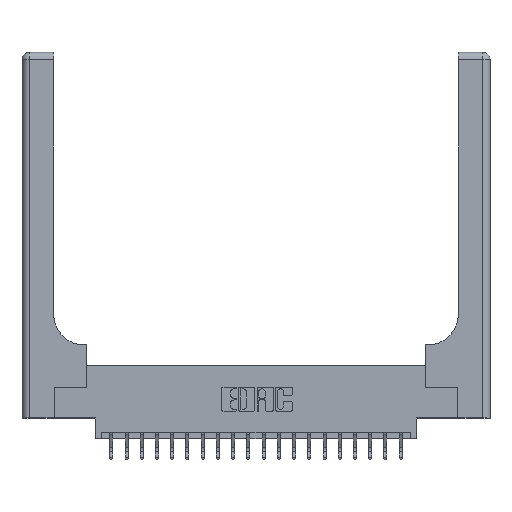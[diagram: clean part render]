
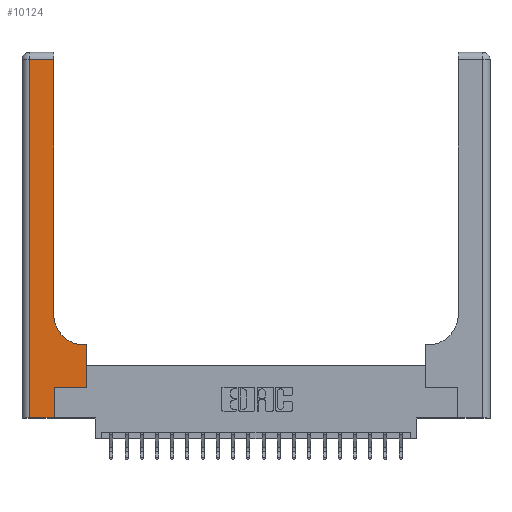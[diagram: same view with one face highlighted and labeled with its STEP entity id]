
A CAD part, top view. The second image highlights one B-rep face of the part: STEP entity #10124.
In plain terms, the highlighted planar face has unit normal (0, 0, 1).
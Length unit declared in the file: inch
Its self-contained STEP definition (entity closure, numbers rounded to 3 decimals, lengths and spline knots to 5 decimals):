
#57 = VERTEX_POINT ( 'NONE', #2765 ) ;
#139 = CARTESIAN_POINT ( 'NONE',  ( 0.528, 0.6, 0.37 ) ) ;
#674 = CIRCLE ( 'NONE', #13136, 0.25 ) ;
#698 = ORIENTED_EDGE ( 'NONE', *, *, #1223, .T. ) ;
#932 = ORIENTED_EDGE ( 'NONE', *, *, #13584, .T. ) ;
#1223 = EDGE_CURVE ( 'NONE', #16627, #3010, #13035, .T. ) ;
#1424 = CARTESIAN_POINT ( 'NONE',  ( 0.26, 0.6, 0.37 ) ) ;
#1683 = CARTESIAN_POINT ( 'NONE',  ( 0.51, 0.85, 0.37 ) ) ;
#1920 = VERTEX_POINT ( 'NONE', #8875 ) ;
#2040 = VECTOR ( 'NONE', #5160, 39.37008 ) ;
#2052 = LINE ( 'NONE', #10752, #2040 ) ;
#2426 = VERTEX_POINT ( 'NONE', #19408 ) ;
#2433 = CARTESIAN_POINT ( 'NONE',  ( 0.265, 0., 0.37 ) ) ;
#2642 = VERTEX_POINT ( 'NONE', #139 ) ;
#2765 = CARTESIAN_POINT ( 'NONE',  ( 0.265, 0., 0.37 ) ) ;
#2771 = ORIENTED_EDGE ( 'NONE', *, *, #15259, .T. ) ;
#2791 = LINE ( 'NONE', #13460, #11475 ) ;
#2866 = LINE ( 'NONE', #1424, #13547 ) ;
#3010 = VERTEX_POINT ( 'NONE', #9829 ) ;
#3106 = EDGE_CURVE ( 'NONE', #17928, #1920, #674, .T. ) ;
#3261 = EDGE_CURVE ( 'NONE', #13300, #2426, #14153, .T. ) ;
#3462 = EDGE_LOOP ( 'NONE', ( #14920, #10365, #698, #2771, #932, #14334, #10957, #6862, #9810 ) ) ;
#4214 = CARTESIAN_POINT ( 'NONE',  ( 0.528, 0.25, 0.37 ) ) ;
#4357 = DIRECTION ( 'NONE',  ( 0., 1., 0. ) ) ;
#4392 = EDGE_CURVE ( 'NONE', #2426, #2642, #17804, .T. ) ;
#5160 = DIRECTION ( 'NONE',  ( -1., 0., 0. ) ) ;
#5792 = DIRECTION ( 'NONE',  ( 0., 1., 0. ) ) ;
#6024 = LINE ( 'NONE', #7929, #8051 ) ;
#6564 = PLANE ( 'NONE',  #13225 ) ;
#6577 = CARTESIAN_POINT ( 'NONE',  ( 0.51, 0.6, 0.37 ) ) ;
#6862 = ORIENTED_EDGE ( 'NONE', *, *, #6983, .T. ) ;
#6983 = EDGE_CURVE ( 'NONE', #2642, #17928, #2866, .T. ) ;
#7684 = DIRECTION ( 'NONE',  ( 1., 0., 0. ) ) ;
#7822 = VECTOR ( 'NONE', #7684, 39.37008 ) ;
#7929 = CARTESIAN_POINT ( 'NONE',  ( 0., 0., 0.37 ) ) ;
#8051 = VECTOR ( 'NONE', #11399, 39.37008 ) ;
#8203 = EDGE_CURVE ( 'NONE', #1920, #18540, #2791, .T. ) ;
#8726 = VECTOR ( 'NONE', #5792, 39.37008 ) ;
#8742 = CARTESIAN_POINT ( 'NONE',  ( 0.26, 2.94, 0.37 ) ) ;
#8875 = CARTESIAN_POINT ( 'NONE',  ( 0.26, 0.85, 0.37 ) ) ;
#9143 = DIRECTION ( 'NONE',  ( 0., 1., 0. ) ) ;
#9810 = ORIENTED_EDGE ( 'NONE', *, *, #3106, .T. ) ;
#9829 = CARTESIAN_POINT ( 'NONE',  ( 0.06, 0., 0.37 ) ) ;
#10124 = ADVANCED_FACE ( 'NONE', ( #15340 ), #6564, .F. ) ;
#10250 = DIRECTION ( 'NONE',  ( 0., 0., -1. ) ) ;
#10365 = ORIENTED_EDGE ( 'NONE', *, *, #18594, .T. ) ;
#10752 = CARTESIAN_POINT ( 'NONE',  ( 0., 2.94, 0.37 ) ) ;
#10957 = ORIENTED_EDGE ( 'NONE', *, *, #4392, .T. ) ;
#11253 = VECTOR ( 'NONE', #9143, 39.37008 ) ;
#11399 = DIRECTION ( 'NONE',  ( 1., 0., 0. ) ) ;
#11475 = VECTOR ( 'NONE', #4357, 39.37008 ) ;
#11596 = DIRECTION ( 'NONE',  ( -1., 0., 0. ) ) ;
#13035 = LINE ( 'NONE', #16474, #18280 ) ;
#13136 = AXIS2_PLACEMENT_3D ( 'NONE', #1683, #13602, #20487 ) ;
#13225 = AXIS2_PLACEMENT_3D ( 'NONE', #13359, #10250, #11596 ) ;
#13300 = VERTEX_POINT ( 'NONE', #18155 ) ;
#13359 = CARTESIAN_POINT ( 'NONE',  ( 0., 3., 0.37 ) ) ;
#13460 = CARTESIAN_POINT ( 'NONE',  ( 0.26, 3., 0.37 ) ) ;
#13547 = VECTOR ( 'NONE', #19792, 39.37008 ) ;
#13584 = EDGE_CURVE ( 'NONE', #57, #13300, #20920, .T. ) ;
#13602 = DIRECTION ( 'NONE',  ( 0., 0., -1. ) ) ;
#14153 = LINE ( 'NONE', #21243, #7822 ) ;
#14334 = ORIENTED_EDGE ( 'NONE', *, *, #3261, .T. ) ;
#14920 = ORIENTED_EDGE ( 'NONE', *, *, #8203, .T. ) ;
#15259 = EDGE_CURVE ( 'NONE', #3010, #57, #6024, .T. ) ;
#15340 = FACE_OUTER_BOUND ( 'NONE', #3462, .T. ) ;
#16409 = CARTESIAN_POINT ( 'NONE',  ( 0.06, 2.94, 0.37 ) ) ;
#16474 = CARTESIAN_POINT ( 'NONE',  ( 0.06, 3., 0.37 ) ) ;
#16627 = VERTEX_POINT ( 'NONE', #16409 ) ;
#17804 = LINE ( 'NONE', #4214, #11253 ) ;
#17928 = VERTEX_POINT ( 'NONE', #6577 ) ;
#18155 = CARTESIAN_POINT ( 'NONE',  ( 0.265, 0.25, 0.37 ) ) ;
#18280 = VECTOR ( 'NONE', #19806, 39.37008 ) ;
#18540 = VERTEX_POINT ( 'NONE', #8742 ) ;
#18594 = EDGE_CURVE ( 'NONE', #18540, #16627, #2052, .T. ) ;
#19408 = CARTESIAN_POINT ( 'NONE',  ( 0.528, 0.25, 0.37 ) ) ;
#19792 = DIRECTION ( 'NONE',  ( -1., 0., 0. ) ) ;
#19806 = DIRECTION ( 'NONE',  ( 0., -1., 0. ) ) ;
#20487 = DIRECTION ( 'NONE',  ( 1., 0., 0. ) ) ;
#20920 = LINE ( 'NONE', #2433, #8726 ) ;
#21243 = CARTESIAN_POINT ( 'NONE',  ( 0.265, 0.25, 0.37 ) ) ;
